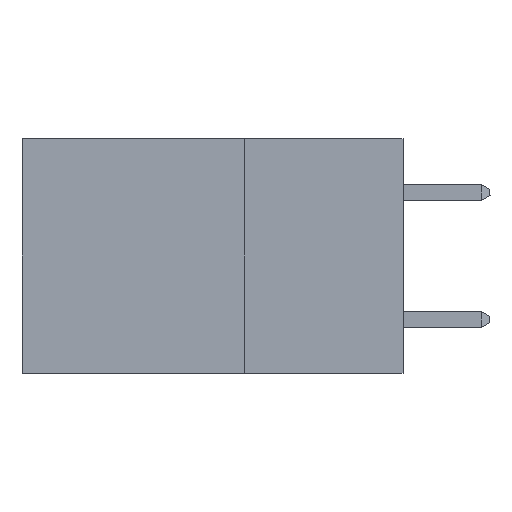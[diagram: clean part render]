
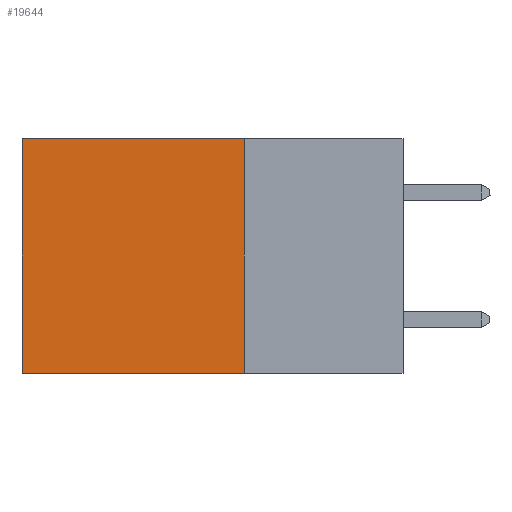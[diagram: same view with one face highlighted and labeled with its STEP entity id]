
A CAD part, left-side view. The second image highlights one B-rep face of the part: STEP entity #19644.
In plain terms, the highlighted planar face has unit normal (-1, 0, 0).
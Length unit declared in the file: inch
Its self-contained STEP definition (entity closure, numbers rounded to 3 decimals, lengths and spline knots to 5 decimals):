
#154 = EDGE_CURVE ( 'NONE', #8346, #4733, #14680, .T. ) ;
#575 = CARTESIAN_POINT ( 'NONE',  ( 0.2875, 0.6, -0.37 ) ) ;
#654 = FACE_OUTER_BOUND ( 'NONE', #19666, .T. ) ;
#1699 = LINE ( 'NONE', #9850, #7055 ) ;
#2405 = ORIENTED_EDGE ( 'NONE', *, *, #6505, .F. ) ;
#3047 = CARTESIAN_POINT ( 'NONE',  ( 0.2875, 0.6, 0. ) ) ;
#3090 = LINE ( 'NONE', #15146, #15610 ) ;
#3103 = CARTESIAN_POINT ( 'NONE',  ( 0.2875, 0.25, -0.37 ) ) ;
#3251 = DIRECTION ( 'NONE',  ( 0., 1., 0. ) ) ;
#3266 = ORIENTED_EDGE ( 'NONE', *, *, #18271, .F. ) ;
#3672 = PLANE ( 'NONE',  #10542 ) ;
#4733 = VERTEX_POINT ( 'NONE', #575 ) ;
#5006 = DIRECTION ( 'NONE',  ( 0., 1., 0. ) ) ;
#5163 = CARTESIAN_POINT ( 'NONE',  ( 0.2875, 0.25, 0. ) ) ;
#6505 = EDGE_CURVE ( 'NONE', #8692, #10958, #3090, .T. ) ;
#6950 = CARTESIAN_POINT ( 'NONE',  ( 0.2875, 0.25, 0. ) ) ;
#7055 = VECTOR ( 'NONE', #5006, 39.37008 ) ;
#7187 = ORIENTED_EDGE ( 'NONE', *, *, #18404, .T. ) ;
#8346 = VERTEX_POINT ( 'NONE', #3047 ) ;
#8692 = VERTEX_POINT ( 'NONE', #5163 ) ;
#8987 = CARTESIAN_POINT ( 'NONE',  ( 0.2875, 0.6, 0. ) ) ;
#9850 = CARTESIAN_POINT ( 'NONE',  ( 0.2875, 0.25, 0. ) ) ;
#10542 = AXIS2_PLACEMENT_3D ( 'NONE', #6950, #11454, #14432 ) ;
#10581 = DIRECTION ( 'NONE',  ( 0., 0., -1. ) ) ;
#10958 = VERTEX_POINT ( 'NONE', #18214 ) ;
#11454 = DIRECTION ( 'NONE',  ( 1., 0., 0. ) ) ;
#11533 = VECTOR ( 'NONE', #10581, 39.37008 ) ;
#14223 = VECTOR ( 'NONE', #3251, 39.37008 ) ;
#14432 = DIRECTION ( 'NONE',  ( 0., 0., -1. ) ) ;
#14680 = LINE ( 'NONE', #8987, #11533 ) ;
#14947 = LINE ( 'NONE', #3103, #14223 ) ;
#15146 = CARTESIAN_POINT ( 'NONE',  ( 0.2875, 0.25, 0. ) ) ;
#15610 = VECTOR ( 'NONE', #16508, 39.37008 ) ;
#16508 = DIRECTION ( 'NONE',  ( 0., 0., -1. ) ) ;
#16835 = ORIENTED_EDGE ( 'NONE', *, *, #154, .T. ) ;
#18214 = CARTESIAN_POINT ( 'NONE',  ( 0.2875, 0.25, -0.37 ) ) ;
#18271 = EDGE_CURVE ( 'NONE', #10958, #4733, #14947, .T. ) ;
#18404 = EDGE_CURVE ( 'NONE', #8692, #8346, #1699, .T. ) ;
#19644 = ADVANCED_FACE ( 'NONE', ( #654 ), #3672, .F. ) ;
#19666 = EDGE_LOOP ( 'NONE', ( #16835, #3266, #2405, #7187 ) ) ;
